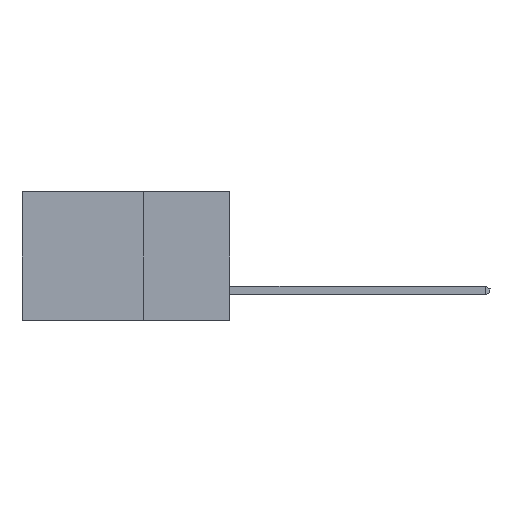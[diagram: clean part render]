
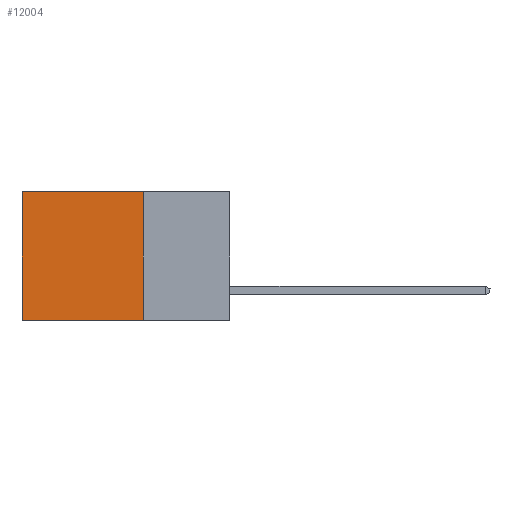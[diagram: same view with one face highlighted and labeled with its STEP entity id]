
A CAD part, left-side view. The second image highlights one B-rep face of the part: STEP entity #12004.
In plain terms, the highlighted planar face has unit normal (-1, 0, 0).
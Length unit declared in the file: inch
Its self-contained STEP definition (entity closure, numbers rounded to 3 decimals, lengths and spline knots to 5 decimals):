
#47 = DIRECTION ( 'NONE',  ( 0., 1., 0. ) ) ;
#141 = CARTESIAN_POINT ( 'NONE',  ( 0.2615, 0.25, -0.37 ) ) ;
#1615 = EDGE_CURVE ( 'NONE', #15068, #6714, #16973, .T. ) ;
#4257 = CARTESIAN_POINT ( 'NONE',  ( 0.2615, 0.25, 0. ) ) ;
#4996 = AXIS2_PLACEMENT_3D ( 'NONE', #141, #11067, #21751 ) ;
#6005 = DIRECTION ( 'NONE',  ( 0., 0., -1. ) ) ;
#6714 = VERTEX_POINT ( 'NONE', #22268 ) ;
#7587 = VECTOR ( 'NONE', #18797, 39.37008 ) ;
#9653 = VECTOR ( 'NONE', #6005, 39.37008 ) ;
#10213 = ORIENTED_EDGE ( 'NONE', *, *, #21261, .F. ) ;
#10851 = CARTESIAN_POINT ( 'NONE',  ( 0.2615, 0.6, 0. ) ) ;
#11067 = DIRECTION ( 'NONE',  ( 1., 0., 0. ) ) ;
#11327 = VERTEX_POINT ( 'NONE', #4257 ) ;
#12004 = ADVANCED_FACE ( 'NONE', ( #21640 ), #12461, .F. ) ;
#12216 = CARTESIAN_POINT ( 'NONE',  ( 0.2615, 0.25, -0.37 ) ) ;
#12461 = PLANE ( 'NONE',  #4996 ) ;
#13366 = EDGE_CURVE ( 'NONE', #11327, #15068, #15157, .T. ) ;
#14033 = EDGE_LOOP ( 'NONE', ( #21275, #10213, #22384, #16994 ) ) ;
#15068 = VERTEX_POINT ( 'NONE', #10851 ) ;
#15157 = LINE ( 'NONE', #19036, #7587 ) ;
#16149 = VERTEX_POINT ( 'NONE', #22123 ) ;
#16945 = EDGE_CURVE ( 'NONE', #11327, #16149, #17524, .T. ) ;
#16973 = LINE ( 'NONE', #18407, #9653 ) ;
#16994 = ORIENTED_EDGE ( 'NONE', *, *, #13366, .T. ) ;
#17524 = LINE ( 'NONE', #12216, #20393 ) ;
#17564 = CARTESIAN_POINT ( 'NONE',  ( 0.2615, 0.25, -0.37 ) ) ;
#18407 = CARTESIAN_POINT ( 'NONE',  ( 0.2615, 0.6, -0.37 ) ) ;
#18797 = DIRECTION ( 'NONE',  ( 0., 1., 0. ) ) ;
#19036 = CARTESIAN_POINT ( 'NONE',  ( 0.2615, 0.25, 0. ) ) ;
#19411 = DIRECTION ( 'NONE',  ( 0., 0., -1. ) ) ;
#20393 = VECTOR ( 'NONE', #19411, 39.37008 ) ;
#21261 = EDGE_CURVE ( 'NONE', #16149, #6714, #23079, .T. ) ;
#21275 = ORIENTED_EDGE ( 'NONE', *, *, #1615, .T. ) ;
#21640 = FACE_OUTER_BOUND ( 'NONE', #14033, .T. ) ;
#21751 = DIRECTION ( 'NONE',  ( 0., 0., -1. ) ) ;
#22123 = CARTESIAN_POINT ( 'NONE',  ( 0.2615, 0.25, -0.37 ) ) ;
#22268 = CARTESIAN_POINT ( 'NONE',  ( 0.2615, 0.6, -0.37 ) ) ;
#22384 = ORIENTED_EDGE ( 'NONE', *, *, #16945, .F. ) ;
#22723 = VECTOR ( 'NONE', #47, 39.37008 ) ;
#23079 = LINE ( 'NONE', #17564, #22723 ) ;
